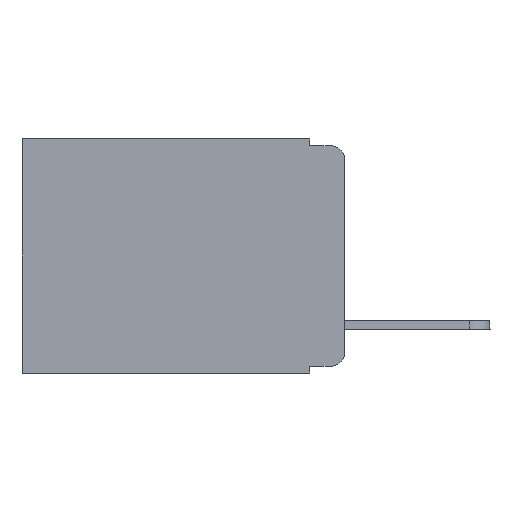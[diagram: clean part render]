
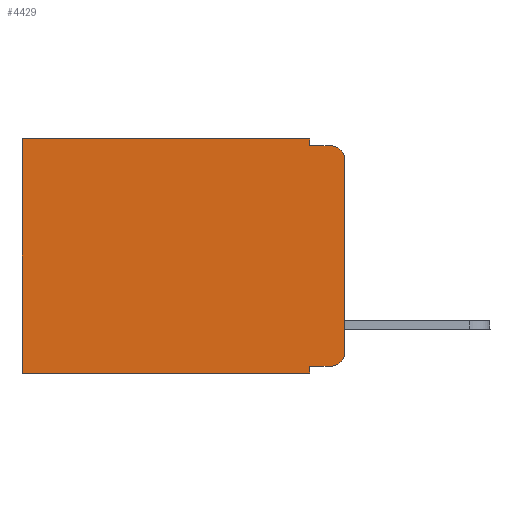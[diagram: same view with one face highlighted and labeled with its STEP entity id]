
A CAD part, left-side view. The second image highlights one B-rep face of the part: STEP entity #4429.
In plain terms, the highlighted planar face has unit normal (-1, 0, 0).
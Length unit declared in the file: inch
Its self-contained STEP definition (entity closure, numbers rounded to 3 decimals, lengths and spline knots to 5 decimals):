
#1 = LINE ( 'NONE', #6502, #7691 ) ;
#242 = CARTESIAN_POINT ( 'NONE',  ( 0.298, 0.473, -0.343 ) ) ;
#565 = EDGE_CURVE ( 'NONE', #9576, #18286, #758, .T. ) ;
#575 = CARTESIAN_POINT ( 'NONE',  ( 0.298, 0.051, -0.343 ) ) ;
#758 = LINE ( 'NONE', #18613, #15456 ) ;
#1016 = CARTESIAN_POINT ( 'NONE',  ( 0.298, 0.02, -0.01 ) ) ;
#1322 = DIRECTION ( 'NONE',  ( 1., 0., 0. ) ) ;
#1415 = ORIENTED_EDGE ( 'NONE', *, *, #6539, .T. ) ;
#1463 = LINE ( 'NONE', #10835, #11650 ) ;
#1766 = CARTESIAN_POINT ( 'NONE',  ( 0.298, 0.02, -0.333 ) ) ;
#1976 = ORIENTED_EDGE ( 'NONE', *, *, #9873, .F. ) ;
#2627 = DIRECTION ( 'NONE',  ( -1., 0., 0. ) ) ;
#2758 = LINE ( 'NONE', #17637, #8981 ) ;
#3387 = EDGE_CURVE ( 'NONE', #19414, #18286, #11960, .T. ) ;
#3389 = ORIENTED_EDGE ( 'NONE', *, *, #11445, .T. ) ;
#3436 = EDGE_CURVE ( 'NONE', #15416, #18128, #13976, .T. ) ;
#3618 = CARTESIAN_POINT ( 'NONE',  ( 0.298, 0., -0.313 ) ) ;
#3936 = CARTESIAN_POINT ( 'NONE',  ( 0.298, 0.02, -0.03 ) ) ;
#4030 = CARTESIAN_POINT ( 'NONE',  ( 0.298, 0.051, 0. ) ) ;
#4429 = ADVANCED_FACE ( 'NONE', ( #4836 ), #9435, .F. ) ;
#4524 = DIRECTION ( 'NONE',  ( 0., 0., -1. ) ) ;
#4629 = VERTEX_POINT ( 'NONE', #242 ) ;
#4836 = FACE_OUTER_BOUND ( 'NONE', #8217, .T. ) ;
#5601 = DIRECTION ( 'NONE',  ( 0., 0., -1. ) ) ;
#5756 = DIRECTION ( 'NONE',  ( 0., 0., -1. ) ) ;
#5821 = CARTESIAN_POINT ( 'NONE',  ( 0.298, 0.473, 0. ) ) ;
#5946 = ORIENTED_EDGE ( 'NONE', *, *, #3436, .T. ) ;
#5978 = DIRECTION ( 'NONE',  ( -1., 0., 0. ) ) ;
#6148 = EDGE_CURVE ( 'NONE', #18662, #4629, #1, .T. ) ;
#6472 = DIRECTION ( 'NONE',  ( 0., 0., -1. ) ) ;
#6502 = CARTESIAN_POINT ( 'NONE',  ( 0.298, 0., -0.343 ) ) ;
#6539 = EDGE_CURVE ( 'NONE', #7372, #17036, #2758, .T. ) ;
#7250 = DIRECTION ( 'NONE',  ( 0., -1., 0. ) ) ;
#7351 = CARTESIAN_POINT ( 'NONE',  ( 0.298, 0.051, -0.01 ) ) ;
#7372 = VERTEX_POINT ( 'NONE', #9514 ) ;
#7614 = AXIS2_PLACEMENT_3D ( 'NONE', #20458, #2627, #18981 ) ;
#7691 = VECTOR ( 'NONE', #15836, 39.37008 ) ;
#7768 = DIRECTION ( 'NONE',  ( 0., 1., 0. ) ) ;
#8162 = VERTEX_POINT ( 'NONE', #3618 ) ;
#8217 = EDGE_LOOP ( 'NONE', ( #1976, #20422, #13066, #21090, #1415, #3389, #8775, #20420, #5946, #17650 ) ) ;
#8325 = VECTOR ( 'NONE', #5756, 39.37008 ) ;
#8775 = ORIENTED_EDGE ( 'NONE', *, *, #6148, .F. ) ;
#8945 = VECTOR ( 'NONE', #5601, 39.37008 ) ;
#8981 = VECTOR ( 'NONE', #7768, 39.37008 ) ;
#9083 = AXIS2_PLACEMENT_3D ( 'NONE', #9749, #1322, #4524 ) ;
#9435 = PLANE ( 'NONE',  #9083 ) ;
#9514 = CARTESIAN_POINT ( 'NONE',  ( 0.298, 0.051, 0. ) ) ;
#9576 = VERTEX_POINT ( 'NONE', #7351 ) ;
#9749 = CARTESIAN_POINT ( 'NONE',  ( 0.298, 0., 0. ) ) ;
#9873 = EDGE_CURVE ( 'NONE', #19414, #8162, #18138, .T. ) ;
#10581 = AXIS2_PLACEMENT_3D ( 'NONE', #3936, #5978, #18598 ) ;
#10594 = CARTESIAN_POINT ( 'NONE',  ( 0.298, 0.051, 0. ) ) ;
#10835 = CARTESIAN_POINT ( 'NONE',  ( 0.298, 0.473, 0. ) ) ;
#11445 = EDGE_CURVE ( 'NONE', #17036, #4629, #1463, .T. ) ;
#11650 = VECTOR ( 'NONE', #17382, 39.37008 ) ;
#11701 = EDGE_CURVE ( 'NONE', #7372, #9576, #11790, .T. ) ;
#11790 = LINE ( 'NONE', #10594, #8945 ) ;
#11960 = CIRCLE ( 'NONE', #10581, 0.02 ) ;
#12500 = EDGE_CURVE ( 'NONE', #18128, #8162, #20231, .T. ) ;
#13066 = ORIENTED_EDGE ( 'NONE', *, *, #565, .F. ) ;
#13321 = VECTOR ( 'NONE', #17403, 39.37008 ) ;
#13674 = EDGE_CURVE ( 'NONE', #15416, #18662, #18473, .T. ) ;
#13976 = LINE ( 'NONE', #20385, #13321 ) ;
#14722 = CARTESIAN_POINT ( 'NONE',  ( 0.298, 0., 0. ) ) ;
#15416 = VERTEX_POINT ( 'NONE', #16637 ) ;
#15456 = VECTOR ( 'NONE', #7250, 39.37008 ) ;
#15836 = DIRECTION ( 'NONE',  ( 0., 1., 0. ) ) ;
#16144 = CARTESIAN_POINT ( 'NONE',  ( 0.298, 0., -0.03 ) ) ;
#16637 = CARTESIAN_POINT ( 'NONE',  ( 0.298, 0.051, -0.333 ) ) ;
#17036 = VERTEX_POINT ( 'NONE', #5821 ) ;
#17382 = DIRECTION ( 'NONE',  ( 0., 0., -1. ) ) ;
#17403 = DIRECTION ( 'NONE',  ( 0., -1., 0. ) ) ;
#17637 = CARTESIAN_POINT ( 'NONE',  ( 0.298, 0., 0. ) ) ;
#17650 = ORIENTED_EDGE ( 'NONE', *, *, #12500, .T. ) ;
#18128 = VERTEX_POINT ( 'NONE', #1766 ) ;
#18138 = LINE ( 'NONE', #14722, #20885 ) ;
#18286 = VERTEX_POINT ( 'NONE', #1016 ) ;
#18473 = LINE ( 'NONE', #4030, #8325 ) ;
#18598 = DIRECTION ( 'NONE',  ( 0., 0., -1. ) ) ;
#18613 = CARTESIAN_POINT ( 'NONE',  ( 0.298, 0.051, -0.01 ) ) ;
#18662 = VERTEX_POINT ( 'NONE', #575 ) ;
#18981 = DIRECTION ( 'NONE',  ( 0., 0., -1. ) ) ;
#19414 = VERTEX_POINT ( 'NONE', #16144 ) ;
#20231 = CIRCLE ( 'NONE', #7614, 0.02 ) ;
#20385 = CARTESIAN_POINT ( 'NONE',  ( 0.298, 0.051, -0.333 ) ) ;
#20420 = ORIENTED_EDGE ( 'NONE', *, *, #13674, .F. ) ;
#20422 = ORIENTED_EDGE ( 'NONE', *, *, #3387, .T. ) ;
#20458 = CARTESIAN_POINT ( 'NONE',  ( 0.298, 0.02, -0.313 ) ) ;
#20885 = VECTOR ( 'NONE', #6472, 39.37008 ) ;
#21090 = ORIENTED_EDGE ( 'NONE', *, *, #11701, .F. ) ;
